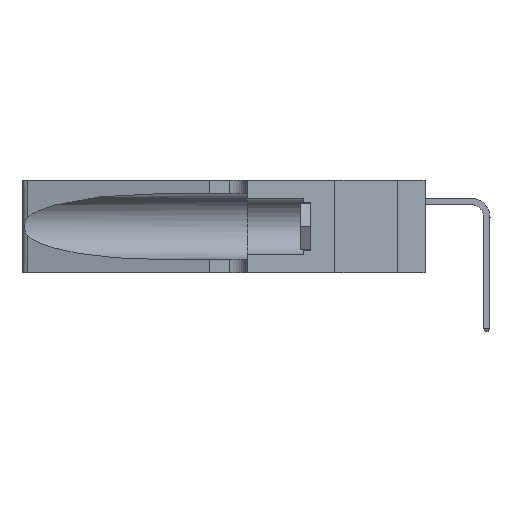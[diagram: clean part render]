
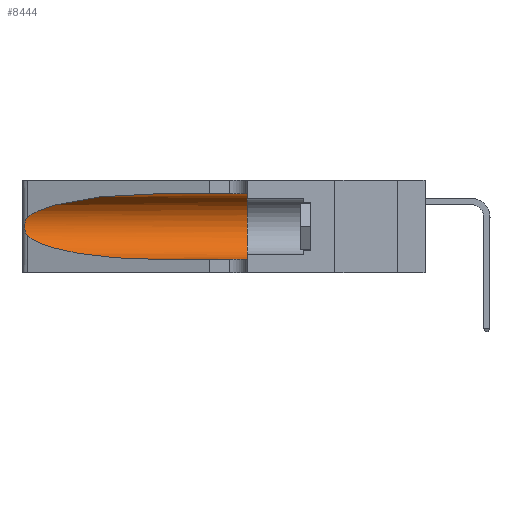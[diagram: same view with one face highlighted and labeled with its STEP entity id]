
A CAD part, left-side view. The second image highlights one B-rep face of the part: STEP entity #8444.
In plain terms, the highlighted cylindrical face has radius 3.308 mm (diameter 6.617 mm), a partial arc.
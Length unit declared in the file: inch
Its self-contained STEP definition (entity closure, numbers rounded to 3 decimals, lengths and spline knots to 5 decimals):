
#298 = ORIENTED_EDGE ( 'NONE', *, *, #20662, .T. ) ;
#306 = EDGE_CURVE ( 'NONE', #6916, #6469, #14297, .T. ) ;
#343 = CARTESIAN_POINT ( 'NONE',  ( 0.1305, 0.72297, 0.05475 ) ) ;
#736 = CARTESIAN_POINT ( 'NONE',  ( 0.25787, 1.23484, 0.2124 ) ) ;
#1400 = VERTEX_POINT ( 'NONE', #16739 ) ;
#1577 = DIRECTION ( 'NONE',  ( 0., -1., 0. ) ) ;
#1606 = B_SPLINE_CURVE_WITH_KNOTS ( 'NONE', 3,
 ( #18305, #2402, #11337, #736, #13110, #2468, #14863, #4248, #16621, #6052, #18389, #7851, #20156, #9647 ),
 .UNSPECIFIED., .F., .F.,
 ( 4, 2, 2, 2, 2, 2, 4 ),
 ( 0., 0.00027, 0.00053, 0.00107, 0.0016, 0.00187, 0.00214 ),
 .UNSPECIFIED. ) ;
#1692 = VERTEX_POINT ( 'NONE', #13752 ) ;
#2005 = DIRECTION ( 'NONE',  ( 0., -1., 0. ) ) ;
#2216 = CARTESIAN_POINT ( 'NONE',  ( 0.2373, 1.15595, 0.08982 ) ) ;
#2402 = CARTESIAN_POINT ( 'NONE',  ( 0.25555, 1.22994, 0.2215 ) ) ;
#2468 = CARTESIAN_POINT ( 'NONE',  ( 0.26018, 1.23835, 0.19895 ) ) ;
#3558 = CARTESIAN_POINT ( 'NONE',  ( 0.2373, 1.15595, 0.28018 ) ) ;
#4248 = CARTESIAN_POINT ( 'NONE',  ( 0.26075, 1.23896, 0.178 ) ) ;
#5297 = VECTOR ( 'NONE', #1577, 39.37008 ) ;
#5360 = CARTESIAN_POINT ( 'NONE',  ( 0.1305, 0.72297, 0.31525 ) ) ;
#5487 = CYLINDRICAL_SURFACE ( 'NONE', #19447, 0.13025 ) ;
#5862 = LINE ( 'NONE', #19075, #5297 ) ;
#6020 = CARTESIAN_POINT ( 'NONE',  ( 0.25487, 1.22718, 0.14631 ) ) ;
#6052 = CARTESIAN_POINT ( 'NONE',  ( 0.25856, 1.23593, 0.16098 ) ) ;
#6100 = CIRCLE ( 'NONE', #7179, 0.13025 ) ;
#6469 = VERTEX_POINT ( 'NONE', #17538 ) ;
#6916 = VERTEX_POINT ( 'NONE', #22302 ) ;
#7179 = AXIS2_PLACEMENT_3D ( 'NONE', #20353, #9835, #22124 ) ;
#7759 = ORIENTED_EDGE ( 'NONE', *, *, #13787, .T. ) ;
#7851 = CARTESIAN_POINT ( 'NONE',  ( 0.25639, 1.23186, 0.15144 ) ) ;
#7852 = DIRECTION ( 'NONE',  ( 0., -1., 0. ) ) ;
#8123 = VECTOR ( 'NONE', #7852, 39.37008 ) ;
#8444 = ADVANCED_FACE ( 'NONE', ( #14897 ), #5487, .F. ) ;
#8708 = LINE ( 'NONE', #13111, #8123 ) ;
#8857 = EDGE_LOOP ( 'NONE', ( #7759, #298, #11183, #18845, #12854, #19133 ) ) ;
#9647 = CARTESIAN_POINT ( 'NONE',  ( 0.25487, 1.22718, 0.14631 ) ) ;
#9835 = DIRECTION ( 'NONE',  ( 0., 1., 0. ) ) ;
#11183 = ORIENTED_EDGE ( 'NONE', *, *, #306, .T. ) ;
#11337 = CARTESIAN_POINT ( 'NONE',  ( 0.25639, 1.23184, 0.21858 ) ) ;
#12092 = CARTESIAN_POINT ( 'NONE',  ( 0.1305, 0.72297, 0.31525 ) ) ;
#12420 = EDGE_CURVE ( 'NONE', #14831, #1692, #5862, .T. ) ;
#12854 = ORIENTED_EDGE ( 'NONE', *, *, #17124, .F. ) ;
#13110 = CARTESIAN_POINT ( 'NONE',  ( 0.25854, 1.2359, 0.20912 ) ) ;
#13111 = CARTESIAN_POINT ( 'NONE',  ( 0.1305, 1.61858, 0.05475 ) ) ;
#13752 = CARTESIAN_POINT ( 'NONE',  ( 0.1305, 0.35, 0.31525 ) ) ;
#13787 = EDGE_CURVE ( 'NONE', #14831, #22347, #16302, .T. ) ;
#14297 =( BOUNDED_CURVE ( )  B_SPLINE_CURVE ( 3, ( #6020, #2216, #17056, #343 ),
 .UNSPECIFIED., .F., .F. ) 
 B_SPLINE_CURVE_WITH_KNOTS ( ( 4, 4 ),
 ( 3.44316, 4.71239 ),
 .UNSPECIFIED. ) 
 CURVE ( )  GEOMETRIC_REPRESENTATION_ITEM ( )  RATIONAL_B_SPLINE_CURVE ( ( 1., 0.87, 0.87, 1. ) ) 
 REPRESENTATION_ITEM ( '' )  );
#14381 = DIRECTION ( 'NONE',  ( 0., 0., -1. ) ) ;
#14831 = VERTEX_POINT ( 'NONE', #12092 ) ;
#14863 = CARTESIAN_POINT ( 'NONE',  ( 0.26075, 1.23896, 0.19203 ) ) ;
#14897 = FACE_OUTER_BOUND ( 'NONE', #8857, .T. ) ;
#15928 = EDGE_CURVE ( 'NONE', #6469, #1400, #8708, .T. ) ;
#15938 = CARTESIAN_POINT ( 'NONE',  ( 0.18966, 0.96281, 0.31525 ) ) ;
#16302 =( BOUNDED_CURVE ( )  B_SPLINE_CURVE ( 3, ( #5360, #15938, #3558, #17690 ),
 .UNSPECIFIED., .F., .F. ) 
 B_SPLINE_CURVE_WITH_KNOTS ( ( 4, 4 ),
 ( 1.5708, 2.84003 ),
 .UNSPECIFIED. ) 
 CURVE ( )  GEOMETRIC_REPRESENTATION_ITEM ( )  RATIONAL_B_SPLINE_CURVE ( ( 1., 0.87, 0.87, 1. ) ) 
 REPRESENTATION_ITEM ( '' )  );
#16621 = CARTESIAN_POINT ( 'NONE',  ( 0.26017, 1.23833, 0.17102 ) ) ;
#16739 = CARTESIAN_POINT ( 'NONE',  ( 0.1305, 0.35, 0.05475 ) ) ;
#17056 = CARTESIAN_POINT ( 'NONE',  ( 0.18966, 0.96281, 0.05475 ) ) ;
#17124 = EDGE_CURVE ( 'NONE', #1692, #1400, #6100, .T. ) ;
#17538 = CARTESIAN_POINT ( 'NONE',  ( 0.1305, 0.72297, 0.05475 ) ) ;
#17690 = CARTESIAN_POINT ( 'NONE',  ( 0.25487, 1.22718, 0.22369 ) ) ;
#18305 = CARTESIAN_POINT ( 'NONE',  ( 0.25487, 1.22718, 0.22369 ) ) ;
#18389 = CARTESIAN_POINT ( 'NONE',  ( 0.25789, 1.23486, 0.15765 ) ) ;
#18845 = ORIENTED_EDGE ( 'NONE', *, *, #15928, .T. ) ;
#19075 = CARTESIAN_POINT ( 'NONE',  ( 0.1305, 1.61858, 0.31525 ) ) ;
#19133 = ORIENTED_EDGE ( 'NONE', *, *, #12420, .F. ) ;
#19447 = AXIS2_PLACEMENT_3D ( 'NONE', #21381, #2005, #14381 ) ;
#20156 = CARTESIAN_POINT ( 'NONE',  ( 0.25555, 1.22993, 0.14849 ) ) ;
#20353 = CARTESIAN_POINT ( 'NONE',  ( 0.1305, 0.35, 0.185 ) ) ;
#20662 = EDGE_CURVE ( 'NONE', #22347, #6916, #1606, .T. ) ;
#21040 = CARTESIAN_POINT ( 'NONE',  ( 0.25487, 1.22718, 0.22369 ) ) ;
#21381 = CARTESIAN_POINT ( 'NONE',  ( 0.1305, 1.61858, 0.185 ) ) ;
#22124 = DIRECTION ( 'NONE',  ( 0., 0., 1. ) ) ;
#22302 = CARTESIAN_POINT ( 'NONE',  ( 0.25487, 1.22718, 0.14631 ) ) ;
#22347 = VERTEX_POINT ( 'NONE', #21040 ) ;
